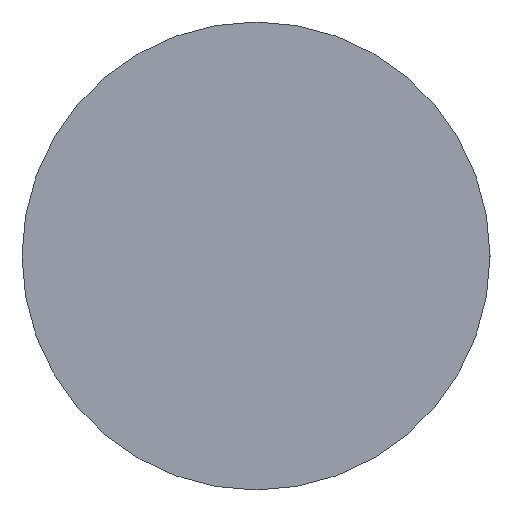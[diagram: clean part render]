
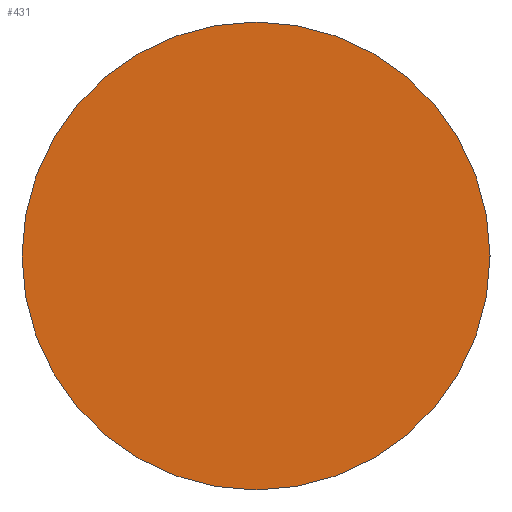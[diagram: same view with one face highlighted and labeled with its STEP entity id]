
A CAD part, left-side view. The second image highlights one B-rep face of the part: STEP entity #431.
In plain terms, the highlighted planar face has unit normal (-1, 0, 0).
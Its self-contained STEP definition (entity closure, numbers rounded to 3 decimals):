
#4 = AXIS2_PLACEMENT_3D ( 'NONE', #241, #622, #56 ) ;
#18 = EDGE_LOOP ( 'NONE', ( #163, #111 ) ) ;
#30 = FACE_OUTER_BOUND ( 'NONE', #18, .T. ) ;
#56 = DIRECTION ( 'NONE',  ( 0., 0., 1. ) ) ;
#111 = ORIENTED_EDGE ( 'NONE', *, *, #335, .T. ) ;
#141 = CARTESIAN_POINT ( 'NONE',  ( -25., 0., 5. ) ) ;
#145 = CARTESIAN_POINT ( 'NONE',  ( -25., 0., 0. ) ) ;
#163 = ORIENTED_EDGE ( 'NONE', *, *, #321, .T. ) ;
#164 = CARTESIAN_POINT ( 'NONE',  ( -25., 0., -5. ) ) ;
#167 = CARTESIAN_POINT ( 'NONE',  ( -25., 0., 0. ) ) ;
#187 = VERTEX_POINT ( 'NONE', #164 ) ;
#220 = DIRECTION ( 'NONE',  ( 0., 0., 1. ) ) ;
#241 = CARTESIAN_POINT ( 'NONE',  ( -25., 0., 0. ) ) ;
#305 = DIRECTION ( 'NONE',  ( 0., 0., -1. ) ) ;
#321 = EDGE_CURVE ( 'NONE', #676, #187, #644, .T. ) ;
#335 = EDGE_CURVE ( 'NONE', #187, #676, #639, .T. ) ;
#401 = PLANE ( 'NONE',  #593 ) ;
#431 = ADVANCED_FACE ( 'NONE', ( #30 ), #401, .F. ) ;
#544 = DIRECTION ( 'NONE',  ( -1., 0., 0. ) ) ;
#550 = AXIS2_PLACEMENT_3D ( 'NONE', #167, #544, #220 ) ;
#593 = AXIS2_PLACEMENT_3D ( 'NONE', #145, #638, #305 ) ;
#622 = DIRECTION ( 'NONE',  ( -1., 0., 0. ) ) ;
#638 = DIRECTION ( 'NONE',  ( 1., 0., 0. ) ) ;
#639 = CIRCLE ( 'NONE', #550, 5. ) ;
#644 = CIRCLE ( 'NONE', #4, 5. ) ;
#676 = VERTEX_POINT ( 'NONE', #141 ) ;
